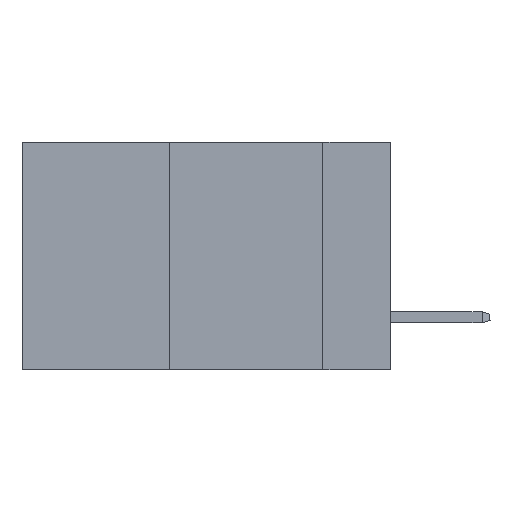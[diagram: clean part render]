
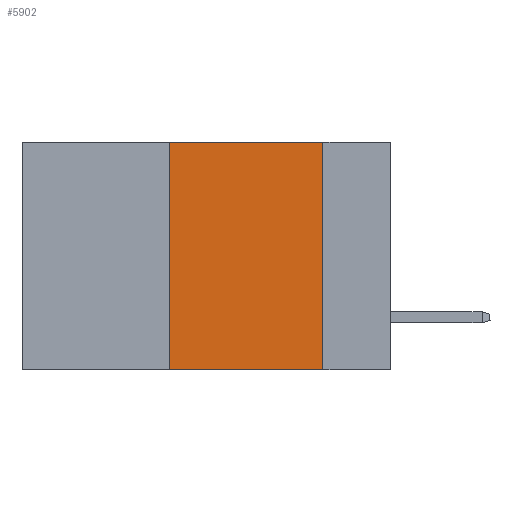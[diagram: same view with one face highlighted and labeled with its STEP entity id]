
A CAD part, left-side view. The second image highlights one B-rep face of the part: STEP entity #5902.
In plain terms, the highlighted planar face has unit normal (-1, 0, 0).
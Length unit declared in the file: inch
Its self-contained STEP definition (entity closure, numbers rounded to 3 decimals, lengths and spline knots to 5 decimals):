
#460 = CARTESIAN_POINT ( 'NONE',  ( 0., 0.36, 0. ) ) ;
#559 = VECTOR ( 'NONE', #4580, 39.37008 ) ;
#714 = FACE_OUTER_BOUND ( 'NONE', #7485, .T. ) ;
#950 = DIRECTION ( 'NONE',  ( 0., 0., -1. ) ) ;
#1005 = VECTOR ( 'NONE', #6333, 39.37008 ) ;
#1615 = VERTEX_POINT ( 'NONE', #5992 ) ;
#3277 = CARTESIAN_POINT ( 'NONE',  ( 0., 0.6, -0.37 ) ) ;
#3313 = ORIENTED_EDGE ( 'NONE', *, *, #11290, .T. ) ;
#3633 = CARTESIAN_POINT ( 'NONE',  ( 0., 0.6, 0. ) ) ;
#4558 = VERTEX_POINT ( 'NONE', #12865 ) ;
#4580 = DIRECTION ( 'NONE',  ( 0., 0., 1. ) ) ;
#4828 = CARTESIAN_POINT ( 'NONE',  ( 0., 0.11, -0.37 ) ) ;
#5271 = CARTESIAN_POINT ( 'NONE',  ( 0., 0.36, -0.37 ) ) ;
#5433 = EDGE_CURVE ( 'NONE', #11044, #1615, #7426, .T. ) ;
#5902 = ADVANCED_FACE ( 'NONE', ( #714 ), #13223, .F. ) ;
#5992 = CARTESIAN_POINT ( 'NONE',  ( 0., 0.36, 0. ) ) ;
#6070 = CARTESIAN_POINT ( 'NONE',  ( 0., 0.11, 0. ) ) ;
#6100 = VECTOR ( 'NONE', #950, 39.37008 ) ;
#6333 = DIRECTION ( 'NONE',  ( 0., -1., 0. ) ) ;
#7098 = DIRECTION ( 'NONE',  ( 1., 0., 0. ) ) ;
#7426 = LINE ( 'NONE', #460, #559 ) ;
#7485 = EDGE_LOOP ( 'NONE', ( #8714, #10742, #12322, #3313 ) ) ;
#7504 = LINE ( 'NONE', #3633, #10883 ) ;
#8269 = DIRECTION ( 'NONE',  ( 0., 0., -1. ) ) ;
#8714 = ORIENTED_EDGE ( 'NONE', *, *, #10718, .F. ) ;
#9022 = LINE ( 'NONE', #6070, #6100 ) ;
#9226 = CARTESIAN_POINT ( 'NONE',  ( 0., 0.6, 0. ) ) ;
#9828 = AXIS2_PLACEMENT_3D ( 'NONE', #9226, #7098, #8269 ) ;
#10718 = EDGE_CURVE ( 'NONE', #4558, #13186, #9022, .T. ) ;
#10742 = ORIENTED_EDGE ( 'NONE', *, *, #13163, .F. ) ;
#10883 = VECTOR ( 'NONE', #11801, 39.37008 ) ;
#11044 = VERTEX_POINT ( 'NONE', #5271 ) ;
#11290 = EDGE_CURVE ( 'NONE', #11044, #13186, #12516, .T. ) ;
#11801 = DIRECTION ( 'NONE',  ( 0., -1., 0. ) ) ;
#12322 = ORIENTED_EDGE ( 'NONE', *, *, #5433, .F. ) ;
#12516 = LINE ( 'NONE', #3277, #1005 ) ;
#12865 = CARTESIAN_POINT ( 'NONE',  ( 0., 0.11, 0. ) ) ;
#13163 = EDGE_CURVE ( 'NONE', #1615, #4558, #7504, .T. ) ;
#13186 = VERTEX_POINT ( 'NONE', #4828 ) ;
#13223 = PLANE ( 'NONE',  #9828 ) ;
